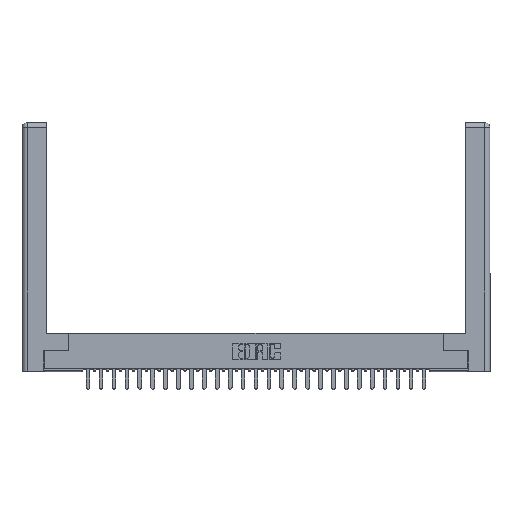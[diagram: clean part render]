
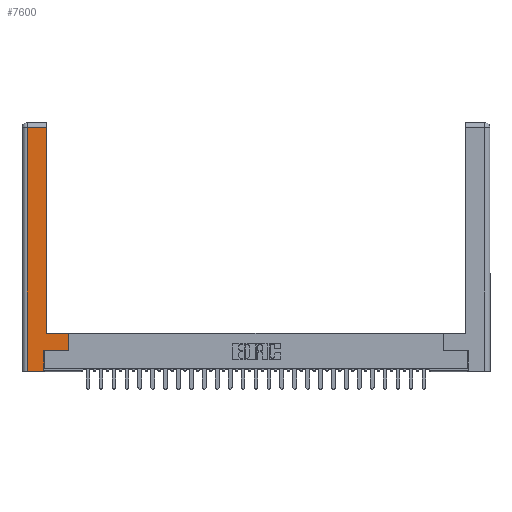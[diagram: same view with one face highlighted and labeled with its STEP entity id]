
A CAD part, top view. The second image highlights one B-rep face of the part: STEP entity #7600.
In plain terms, the highlighted planar face has unit normal (0, 0, 1).
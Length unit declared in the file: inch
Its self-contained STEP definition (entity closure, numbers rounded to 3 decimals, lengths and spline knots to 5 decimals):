
#116 = EDGE_CURVE ( 'NONE', #19648, #29507, #2738, .T. ) ;
#192 = ORIENTED_EDGE ( 'NONE', *, *, #116, .T. ) ;
#1164 = VERTEX_POINT ( 'NONE', #16790 ) ;
#1384 = VERTEX_POINT ( 'NONE', #11543 ) ;
#2141 = VECTOR ( 'NONE', #32184, 39.37008 ) ;
#2250 = DIRECTION ( 'NONE',  ( 0., -1., 0. ) ) ;
#2738 = LINE ( 'NONE', #9581, #29533 ) ;
#3289 = DIRECTION ( 'NONE',  ( -1., 0., 0. ) ) ;
#3558 = ORIENTED_EDGE ( 'NONE', *, *, #8204, .T. ) ;
#4362 = LINE ( 'NONE', #25632, #10835 ) ;
#5083 = EDGE_CURVE ( 'NONE', #14624, #18623, #7783, .T. ) ;
#5826 = ORIENTED_EDGE ( 'NONE', *, *, #25544, .T. ) ;
#6554 = ORIENTED_EDGE ( 'NONE', *, *, #12216, .T. ) ;
#6728 = CARTESIAN_POINT ( 'NONE',  ( 0.0615, 2.94, 0. ) ) ;
#7120 = DIRECTION ( 'NONE',  ( 1., 0., 0. ) ) ;
#7600 = ADVANCED_FACE ( 'NONE', ( #17209 ), #28307, .F. ) ;
#7771 = DIRECTION ( 'NONE',  ( 0., 1., 0. ) ) ;
#7783 = LINE ( 'NONE', #10574, #21644 ) ;
#8079 = EDGE_CURVE ( 'NONE', #18623, #1384, #24880, .T. ) ;
#8204 = EDGE_CURVE ( 'NONE', #29507, #25176, #24450, .T. ) ;
#9581 = CARTESIAN_POINT ( 'NONE',  ( 0.0615, 0., 0. ) ) ;
#9752 = CARTESIAN_POINT ( 'NONE',  ( 0.295, 3., 0. ) ) ;
#9819 = CARTESIAN_POINT ( 'NONE',  ( 0.565, 0.245, 0. ) ) ;
#9863 = DIRECTION ( 'NONE',  ( 0., 1., 0. ) ) ;
#10547 = EDGE_CURVE ( 'NONE', #25176, #30889, #4362, .T. ) ;
#10574 = CARTESIAN_POINT ( 'NONE',  ( 0.295, 0.45, 0. ) ) ;
#10835 = VECTOR ( 'NONE', #7771, 39.37008 ) ;
#10947 = CARTESIAN_POINT ( 'NONE',  ( 0.265, 0., 0. ) ) ;
#11445 = CARTESIAN_POINT ( 'NONE',  ( 0.295, 0.45, 0. ) ) ;
#11543 = CARTESIAN_POINT ( 'NONE',  ( 0.295, 2.94, 0. ) ) ;
#12091 = EDGE_LOOP ( 'NONE', ( #32056, #6554, #192, #3558, #31660, #30594, #5826, #24927 ) ) ;
#12216 = EDGE_CURVE ( 'NONE', #1384, #19648, #33502, .T. ) ;
#12696 = VECTOR ( 'NONE', #9863, 39.37008 ) ;
#12721 = CARTESIAN_POINT ( 'NONE',  ( 0.565, 0.45, 0. ) ) ;
#13074 = DIRECTION ( 'NONE',  ( -1., 0., 0. ) ) ;
#14624 = VERTEX_POINT ( 'NONE', #12721 ) ;
#16671 = LINE ( 'NONE', #9819, #23971 ) ;
#16790 = CARTESIAN_POINT ( 'NONE',  ( 0.565, 0.245, 0. ) ) ;
#17209 = FACE_OUTER_BOUND ( 'NONE', #12091, .T. ) ;
#17550 = CARTESIAN_POINT ( 'NONE',  ( 0.265, 0., 0. ) ) ;
#17589 = EDGE_CURVE ( 'NONE', #30889, #1164, #16671, .T. ) ;
#18623 = VERTEX_POINT ( 'NONE', #11445 ) ;
#18804 = CARTESIAN_POINT ( 'NONE',  ( 0.0615, 0., 0. ) ) ;
#19648 = VERTEX_POINT ( 'NONE', #6728 ) ;
#19877 = AXIS2_PLACEMENT_3D ( 'NONE', #20299, #20515, #33288 ) ;
#20299 = CARTESIAN_POINT ( 'NONE',  ( 0., 0., 0. ) ) ;
#20515 = DIRECTION ( 'NONE',  ( 0., 0., -1. ) ) ;
#20948 = VECTOR ( 'NONE', #3289, 39.37008 ) ;
#21644 = VECTOR ( 'NONE', #13074, 39.37008 ) ;
#23184 = VECTOR ( 'NONE', #24411, 39.37008 ) ;
#23971 = VECTOR ( 'NONE', #7120, 39.37008 ) ;
#24411 = DIRECTION ( 'NONE',  ( 0., 1., 0. ) ) ;
#24450 = LINE ( 'NONE', #10947, #2141 ) ;
#24880 = LINE ( 'NONE', #9752, #12696 ) ;
#24927 = ORIENTED_EDGE ( 'NONE', *, *, #5083, .T. ) ;
#25176 = VERTEX_POINT ( 'NONE', #17550 ) ;
#25544 = EDGE_CURVE ( 'NONE', #1164, #14624, #33314, .T. ) ;
#25632 = CARTESIAN_POINT ( 'NONE',  ( 0.265, 0.245, 0. ) ) ;
#26661 = CARTESIAN_POINT ( 'NONE',  ( 0.565, 0.45, 0. ) ) ;
#28307 = PLANE ( 'NONE',  #19877 ) ;
#29365 = CARTESIAN_POINT ( 'NONE',  ( 0.0615, 2.94, 0. ) ) ;
#29507 = VERTEX_POINT ( 'NONE', #18804 ) ;
#29533 = VECTOR ( 'NONE', #2250, 39.37008 ) ;
#30384 = CARTESIAN_POINT ( 'NONE',  ( 0.265, 0.245, 0. ) ) ;
#30594 = ORIENTED_EDGE ( 'NONE', *, *, #17589, .T. ) ;
#30889 = VERTEX_POINT ( 'NONE', #30384 ) ;
#31660 = ORIENTED_EDGE ( 'NONE', *, *, #10547, .T. ) ;
#32056 = ORIENTED_EDGE ( 'NONE', *, *, #8079, .T. ) ;
#32184 = DIRECTION ( 'NONE',  ( 1., 0., 0. ) ) ;
#33288 = DIRECTION ( 'NONE',  ( -1., 0., 0. ) ) ;
#33314 = LINE ( 'NONE', #26661, #23184 ) ;
#33502 = LINE ( 'NONE', #29365, #20948 ) ;
